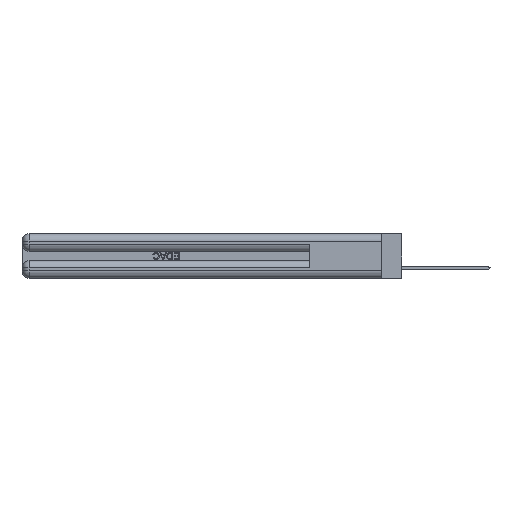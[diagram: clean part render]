
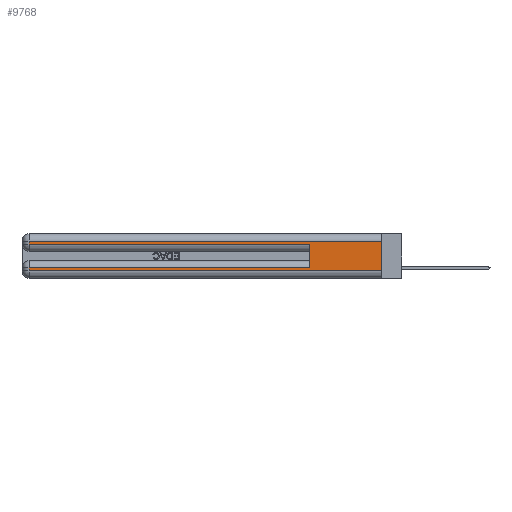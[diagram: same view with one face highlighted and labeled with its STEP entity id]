
A CAD part, left-side view. The second image highlights one B-rep face of the part: STEP entity #9768.
In plain terms, the highlighted planar face has unit normal (-1, 0, 0).
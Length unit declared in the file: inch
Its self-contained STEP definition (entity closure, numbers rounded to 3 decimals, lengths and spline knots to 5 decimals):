
#217 = VECTOR ( 'NONE', #23649, 39.37008 ) ;
#230 = VECTOR ( 'NONE', #36722, 39.37008 ) ;
#665 = VECTOR ( 'NONE', #21967, 39.37008 ) ;
#707 = VERTEX_POINT ( 'NONE', #33706 ) ;
#1018 = DIRECTION ( 'NONE',  ( 0., -1., 0. ) ) ;
#2702 = LINE ( 'NONE', #6682, #217 ) ;
#4541 = EDGE_CURVE ( 'NONE', #23944, #46438, #14348, .T. ) ;
#4684 = VERTEX_POINT ( 'NONE', #15406 ) ;
#5401 = DIRECTION ( 'NONE',  ( 0., 0., -1. ) ) ;
#5759 = CARTESIAN_POINT ( 'NONE',  ( 0., 2.94, 0.37 ) ) ;
#6375 = CARTESIAN_POINT ( 'NONE',  ( 0., 2.94, 0.37 ) ) ;
#6682 = CARTESIAN_POINT ( 'NONE',  ( 0., 0., 0.37 ) ) ;
#8243 = AXIS2_PLACEMENT_3D ( 'NONE', #45437, #10095, #49456 ) ;
#8616 = VECTOR ( 'NONE', #14709, 39.37008 ) ;
#8825 = CARTESIAN_POINT ( 'NONE',  ( 0., 0., 0.285 ) ) ;
#9768 = ADVANCED_FACE ( 'NONE', ( #25208 ), #29353, .F. ) ;
#10095 = DIRECTION ( 'NONE',  ( 1., 0., 0. ) ) ;
#10133 = VECTOR ( 'NONE', #14519, 39.37008 ) ;
#11361 = VERTEX_POINT ( 'NONE', #20903 ) ;
#12662 = EDGE_CURVE ( 'NONE', #707, #38684, #40574, .T. ) ;
#14119 = EDGE_CURVE ( 'NONE', #4684, #38684, #2702, .T. ) ;
#14348 = LINE ( 'NONE', #29818, #665 ) ;
#14519 = DIRECTION ( 'NONE',  ( 0., -1., 0. ) ) ;
#14709 = DIRECTION ( 'NONE',  ( 0., 0., -1. ) ) ;
#15406 = CARTESIAN_POINT ( 'NONE',  ( 0., 0., 0.31 ) ) ;
#15733 = VERTEX_POINT ( 'NONE', #49652 ) ;
#16986 = LINE ( 'NONE', #17044, #230 ) ;
#17044 = CARTESIAN_POINT ( 'NONE',  ( 0., 0., 0.31 ) ) ;
#17055 = ORIENTED_EDGE ( 'NONE', *, *, #48273, .T. ) ;
#18477 = VECTOR ( 'NONE', #28654, 39.37008 ) ;
#19066 = ORIENTED_EDGE ( 'NONE', *, *, #4541, .F. ) ;
#20903 = CARTESIAN_POINT ( 'NONE',  ( 0., 2.94, 0.285 ) ) ;
#21410 = CARTESIAN_POINT ( 'NONE',  ( 0., 0., 0.06 ) ) ;
#21530 = ORIENTED_EDGE ( 'NONE', *, *, #14119, .F. ) ;
#21967 = DIRECTION ( 'NONE',  ( 0., 0., 1. ) ) ;
#22895 = CARTESIAN_POINT ( 'NONE',  ( 0., 0.6, 0.285 ) ) ;
#23103 = EDGE_CURVE ( 'NONE', #48673, #11361, #37340, .T. ) ;
#23649 = DIRECTION ( 'NONE',  ( 0., 0., -1. ) ) ;
#23855 = EDGE_CURVE ( 'NONE', #15733, #707, #29139, .T. ) ;
#23944 = VERTEX_POINT ( 'NONE', #26422 ) ;
#24642 = LINE ( 'NONE', #44569, #18477 ) ;
#25208 = FACE_OUTER_BOUND ( 'NONE', #39090, .T. ) ;
#26422 = CARTESIAN_POINT ( 'NONE',  ( 0., 0.6, 0.085 ) ) ;
#27543 = ORIENTED_EDGE ( 'NONE', *, *, #46130, .T. ) ;
#27603 = EDGE_CURVE ( 'NONE', #23944, #15733, #24642, .T. ) ;
#28654 = DIRECTION ( 'NONE',  ( 0., 1., 0. ) ) ;
#29139 = LINE ( 'NONE', #5759, #49171 ) ;
#29353 = PLANE ( 'NONE',  #8243 ) ;
#29818 = CARTESIAN_POINT ( 'NONE',  ( 0., 0.6, 0.145 ) ) ;
#31183 = ORIENTED_EDGE ( 'NONE', *, *, #23103, .T. ) ;
#31489 = ORIENTED_EDGE ( 'NONE', *, *, #23855, .T. ) ;
#32054 = ORIENTED_EDGE ( 'NONE', *, *, #27603, .T. ) ;
#33706 = CARTESIAN_POINT ( 'NONE',  ( 0., 2.94, 0.06 ) ) ;
#35983 = CARTESIAN_POINT ( 'NONE',  ( 0., 2.94, 0.31 ) ) ;
#36722 = DIRECTION ( 'NONE',  ( 0., 1., 0. ) ) ;
#37340 = LINE ( 'NONE', #6375, #8616 ) ;
#38684 = VERTEX_POINT ( 'NONE', #47068 ) ;
#39090 = EDGE_LOOP ( 'NONE', ( #21530, #17055, #31183, #27543, #19066, #32054, #31489, #47796 ) ) ;
#40170 = LINE ( 'NONE', #8825, #50288 ) ;
#40574 = LINE ( 'NONE', #21410, #10133 ) ;
#44569 = CARTESIAN_POINT ( 'NONE',  ( 0., 0., 0.085 ) ) ;
#45437 = CARTESIAN_POINT ( 'NONE',  ( 0., 0., 0.37 ) ) ;
#46130 = EDGE_CURVE ( 'NONE', #11361, #46438, #40170, .T. ) ;
#46438 = VERTEX_POINT ( 'NONE', #22895 ) ;
#47068 = CARTESIAN_POINT ( 'NONE',  ( 0., 0., 0.06 ) ) ;
#47796 = ORIENTED_EDGE ( 'NONE', *, *, #12662, .T. ) ;
#48273 = EDGE_CURVE ( 'NONE', #4684, #48673, #16986, .T. ) ;
#48673 = VERTEX_POINT ( 'NONE', #35983 ) ;
#49171 = VECTOR ( 'NONE', #5401, 39.37008 ) ;
#49456 = DIRECTION ( 'NONE',  ( 0., 0., -1. ) ) ;
#49652 = CARTESIAN_POINT ( 'NONE',  ( 0., 2.94, 0.085 ) ) ;
#50288 = VECTOR ( 'NONE', #1018, 39.37008 ) ;
